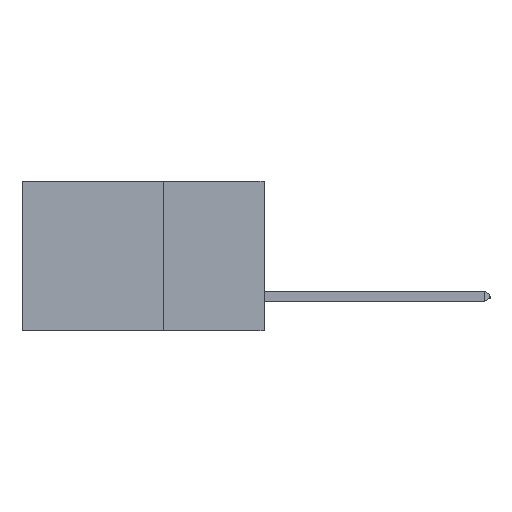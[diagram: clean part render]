
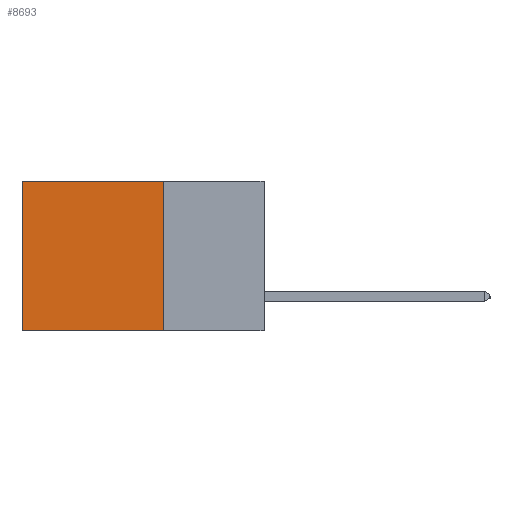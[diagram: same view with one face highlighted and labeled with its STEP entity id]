
A CAD part, left-side view. The second image highlights one B-rep face of the part: STEP entity #8693.
In plain terms, the highlighted planar face has unit normal (-1, 0, 0).
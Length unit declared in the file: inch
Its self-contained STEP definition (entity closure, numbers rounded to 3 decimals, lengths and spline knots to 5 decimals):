
#358 = VERTEX_POINT ( 'NONE', #5455 ) ;
#1095 = LINE ( 'NONE', #3065, #7351 ) ;
#1106 = DIRECTION ( 'NONE',  ( 1., 0., 0. ) ) ;
#1915 = ORIENTED_EDGE ( 'NONE', *, *, #10370, .F. ) ;
#2532 = VECTOR ( 'NONE', #5981, 39.37008 ) ;
#3065 = CARTESIAN_POINT ( 'NONE',  ( 0.298, 0.25, 0. ) ) ;
#3293 = ORIENTED_EDGE ( 'NONE', *, *, #4988, .T. ) ;
#3362 = CARTESIAN_POINT ( 'NONE',  ( 0.298, 0.6, 0. ) ) ;
#3530 = VERTEX_POINT ( 'NONE', #5109 ) ;
#4175 = DIRECTION ( 'NONE',  ( 0., 0., -1. ) ) ;
#4181 = LINE ( 'NONE', #6390, #2532 ) ;
#4368 = CARTESIAN_POINT ( 'NONE',  ( 0.298, 0.25, 0. ) ) ;
#4406 = DIRECTION ( 'NONE',  ( 0., 0., -1. ) ) ;
#4585 = VERTEX_POINT ( 'NONE', #8152 ) ;
#4737 = EDGE_LOOP ( 'NONE', ( #7193, #7946, #1915, #3293 ) ) ;
#4988 = EDGE_CURVE ( 'NONE', #358, #10227, #1095, .T. ) ;
#5041 = CARTESIAN_POINT ( 'NONE',  ( 0.298, 0.6, 0. ) ) ;
#5109 = CARTESIAN_POINT ( 'NONE',  ( 0.298, 0.6, -0.37 ) ) ;
#5148 = LINE ( 'NONE', #3362, #7574 ) ;
#5455 = CARTESIAN_POINT ( 'NONE',  ( 0.298, 0.25, 0. ) ) ;
#5682 = DIRECTION ( 'NONE',  ( 0., 1., 0. ) ) ;
#5819 = EDGE_CURVE ( 'NONE', #4585, #3530, #4181, .T. ) ;
#5981 = DIRECTION ( 'NONE',  ( 0., 1., 0. ) ) ;
#6007 = PLANE ( 'NONE',  #8750 ) ;
#6390 = CARTESIAN_POINT ( 'NONE',  ( 0.298, 0.25, -0.37 ) ) ;
#6831 = DIRECTION ( 'NONE',  ( 0., 0., -1. ) ) ;
#6867 = CARTESIAN_POINT ( 'NONE',  ( 0.298, 0.25, 0. ) ) ;
#6920 = LINE ( 'NONE', #6867, #7160 ) ;
#7160 = VECTOR ( 'NONE', #4406, 39.37008 ) ;
#7193 = ORIENTED_EDGE ( 'NONE', *, *, #9733, .T. ) ;
#7351 = VECTOR ( 'NONE', #5682, 39.37008 ) ;
#7574 = VECTOR ( 'NONE', #4175, 39.37008 ) ;
#7946 = ORIENTED_EDGE ( 'NONE', *, *, #5819, .F. ) ;
#8152 = CARTESIAN_POINT ( 'NONE',  ( 0.298, 0.25, -0.37 ) ) ;
#8693 = ADVANCED_FACE ( 'NONE', ( #8933 ), #6007, .F. ) ;
#8750 = AXIS2_PLACEMENT_3D ( 'NONE', #4368, #1106, #6831 ) ;
#8933 = FACE_OUTER_BOUND ( 'NONE', #4737, .T. ) ;
#9733 = EDGE_CURVE ( 'NONE', #10227, #3530, #5148, .T. ) ;
#10227 = VERTEX_POINT ( 'NONE', #5041 ) ;
#10370 = EDGE_CURVE ( 'NONE', #358, #4585, #6920, .T. ) ;
